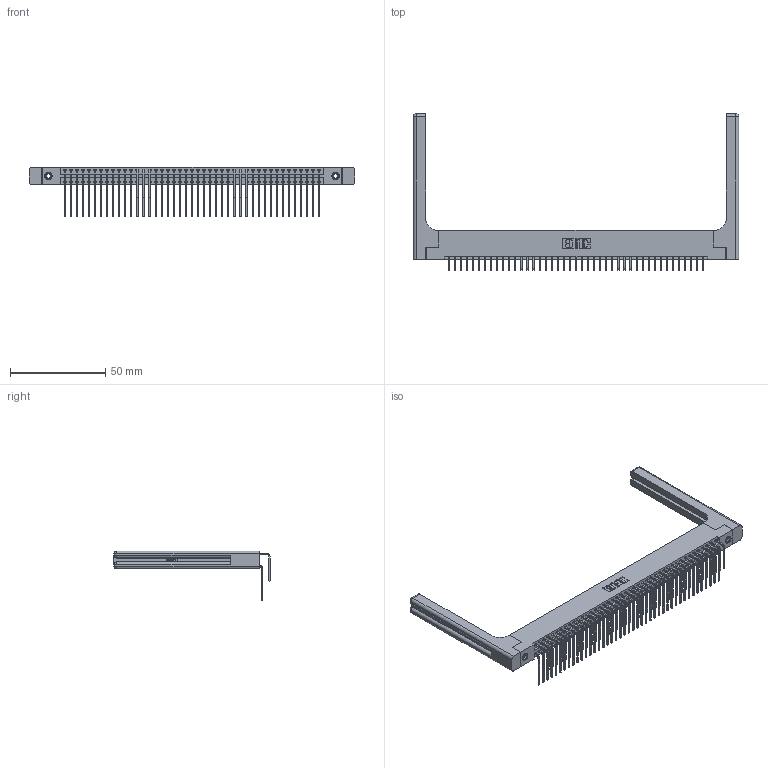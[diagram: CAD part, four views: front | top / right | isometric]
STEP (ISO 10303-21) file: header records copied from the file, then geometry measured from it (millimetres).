
FILE_DESCRIPTION (( 'STEP AP203' ), '1' );
FILE_NAME ('346-086-559-258.STEP', '2022-05-25T23:36:40', ( '' ), ( '' ), 'SwSTEP 2.0', 'SolidWorks 2020', '' );
FILE_SCHEMA (( 'CONFIG_CONTROL_DESIGN' ));
Length unit declared in the file: inch
Products named in the file (6): 345-292-001_559 Tail - 2; 345-250-001_345-250-001-102; 346-220-058_345-220-058; 346 Part_Flush Mounting Lugs - 0.156 Dia-TH; 346-086-559-258; 345-292-001_558 559 Tail - 1
Assembly tree (91 placements, depth 2):
  346-086-559-258
    346 Part_Flush Mounting Lugs - 0.156 Dia-TH
    345-292-001_558 559 Tail - 1  x43
    345-292-001_559 Tail - 2  x43
    345-250-001_345-250-001-102  x2
    346-220-058_345-220-058  x2
Bounding box: 170.59 x 81.85 x 26.16 mm (x, y, z)
Volume: 24614.3 mm3; surface area: 30935.8 mm2
Topology: 91 solids, 91 shells, 5036 faces, 14877 edges, 9782 vertices
Faces by surface type: plane 3420, cylinder 1556, bspline 36, cone 12, sphere 8, torus 4
Entity records: 35310 total; most frequent: CARTESIAN_POINT 6882, ORIENTED_EDGE 5560, DIRECTION 5020, EDGE_CURVE 2780, LINE 2344, VECTOR 2344, VERTEX_POINT 1842, AXIS2_PLACEMENT_3D 1338
